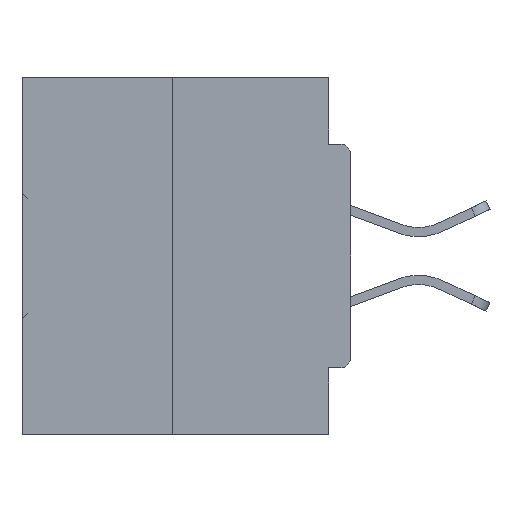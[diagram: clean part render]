
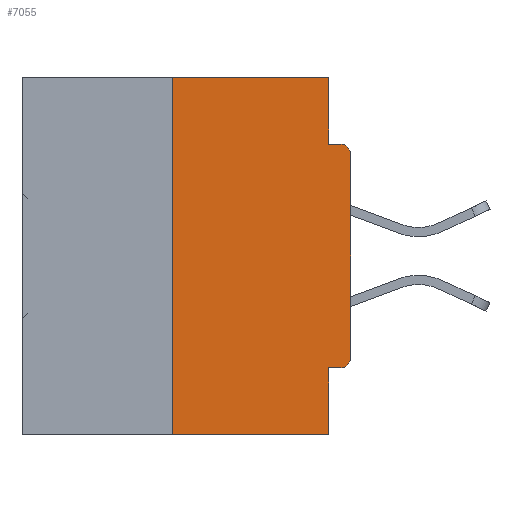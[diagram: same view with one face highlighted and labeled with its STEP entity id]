
A CAD part, left-side view. The second image highlights one B-rep face of the part: STEP entity #7055.
In plain terms, the highlighted planar face has unit normal (-1, 0, 0).
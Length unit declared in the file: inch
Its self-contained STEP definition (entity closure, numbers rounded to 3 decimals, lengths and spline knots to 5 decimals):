
#1575 = VECTOR ( 'NONE', #18556, 39.37008 ) ;
#1924 = DIRECTION ( 'NONE',  ( 0., -1., 0. ) ) ;
#2705 = CARTESIAN_POINT ( 'NONE',  ( 0., 0., 0. ) ) ;
#3144 = VERTEX_POINT ( 'NONE', #39495 ) ;
#3429 = DIRECTION ( 'NONE',  ( -1., 0., 0. ) ) ;
#3908 = EDGE_CURVE ( 'NONE', #16552, #6881, #36625, .T. ) ;
#4827 = VECTOR ( 'NONE', #1924, 39.37008 ) ;
#5094 = ORIENTED_EDGE ( 'NONE', *, *, #28086, .F. ) ;
#5101 = LINE ( 'NONE', #40696, #1575 ) ;
#6521 = VECTOR ( 'NONE', #32120, 39.37008 ) ;
#6881 = VERTEX_POINT ( 'NONE', #27274 ) ;
#7055 = ADVANCED_FACE ( 'NONE', ( #13979 ), #13482, .F. ) ;
#7340 = VECTOR ( 'NONE', #43038, 39.37008 ) ;
#7784 = CARTESIAN_POINT ( 'NONE',  ( 0., 0.015, -0.0935 ) ) ;
#8448 = LINE ( 'NONE', #17828, #7340 ) ;
#8739 = VERTEX_POINT ( 'NONE', #44485 ) ;
#9633 = CARTESIAN_POINT ( 'NONE',  ( 0., 0.46, 0. ) ) ;
#10020 = EDGE_CURVE ( 'NONE', #11931, #46779, #8448, .T. ) ;
#10281 = ORIENTED_EDGE ( 'NONE', *, *, #3908, .T. ) ;
#10805 = EDGE_CURVE ( 'NONE', #3144, #16552, #19893, .T. ) ;
#11190 = CARTESIAN_POINT ( 'NONE',  ( 0., 0.031, -0.5 ) ) ;
#11375 = ORIENTED_EDGE ( 'NONE', *, *, #41169, .F. ) ;
#11489 = EDGE_CURVE ( 'NONE', #29229, #46779, #35936, .T. ) ;
#11931 = VERTEX_POINT ( 'NONE', #34386 ) ;
#13482 = PLANE ( 'NONE',  #47534 ) ;
#13979 = FACE_OUTER_BOUND ( 'NONE', #43682, .T. ) ;
#15105 = CARTESIAN_POINT ( 'NONE',  ( 0., 0.031, -0.5 ) ) ;
#15498 = CARTESIAN_POINT ( 'NONE',  ( 0., 0.015, -0.1085 ) ) ;
#16552 = VERTEX_POINT ( 'NONE', #32540 ) ;
#17175 = DIRECTION ( 'NONE',  ( 1., 0., 0. ) ) ;
#17579 = ORIENTED_EDGE ( 'NONE', *, *, #40966, .F. ) ;
#17828 = CARTESIAN_POINT ( 'NONE',  ( 0., 0.46, -0.5 ) ) ;
#18556 = DIRECTION ( 'NONE',  ( 0., 1., 0. ) ) ;
#18676 = EDGE_CURVE ( 'NONE', #11931, #27597, #25177, .T. ) ;
#19254 = CARTESIAN_POINT ( 'NONE',  ( 0., 0.25, 0. ) ) ;
#19893 = CIRCLE ( 'NONE', #26621, 0.015 ) ;
#20139 = CIRCLE ( 'NONE', #34508, 0.015 ) ;
#20287 = VECTOR ( 'NONE', #37234, 39.37008 ) ;
#23062 = DIRECTION ( 'NONE',  ( 0., 0., -1. ) ) ;
#24182 = EDGE_CURVE ( 'NONE', #6881, #32435, #20139, .T. ) ;
#25177 = LINE ( 'NONE', #41457, #40215 ) ;
#25526 = CARTESIAN_POINT ( 'NONE',  ( 0., 0.015, -0.3915 ) ) ;
#26477 = DIRECTION ( 'NONE',  ( -1., 0., 0. ) ) ;
#26621 = AXIS2_PLACEMENT_3D ( 'NONE', #25526, #3429, #40404 ) ;
#26724 = DIRECTION ( 'NONE',  ( 0., 0., 1. ) ) ;
#27274 = CARTESIAN_POINT ( 'NONE',  ( 0., 0., -0.1085 ) ) ;
#27381 = VERTEX_POINT ( 'NONE', #32079 ) ;
#27597 = VERTEX_POINT ( 'NONE', #19254 ) ;
#28077 = CARTESIAN_POINT ( 'NONE',  ( 0., 0., -0.0935 ) ) ;
#28086 = EDGE_CURVE ( 'NONE', #27597, #8739, #30184, .T. ) ;
#29229 = VERTEX_POINT ( 'NONE', #33260 ) ;
#29304 = VECTOR ( 'NONE', #37919, 39.37008 ) ;
#30184 = LINE ( 'NONE', #42281, #4827 ) ;
#31139 = ORIENTED_EDGE ( 'NONE', *, *, #10805, .T. ) ;
#32079 = CARTESIAN_POINT ( 'NONE',  ( 0., 0.031, -0.0935 ) ) ;
#32120 = DIRECTION ( 'NONE',  ( 0., -1., 0. ) ) ;
#32435 = VERTEX_POINT ( 'NONE', #7784 ) ;
#32540 = CARTESIAN_POINT ( 'NONE',  ( 0., 0., -0.3915 ) ) ;
#33260 = CARTESIAN_POINT ( 'NONE',  ( 0., 0.031, -0.4065 ) ) ;
#33725 = VECTOR ( 'NONE', #36132, 39.37008 ) ;
#34386 = CARTESIAN_POINT ( 'NONE',  ( 0., 0.25, -0.5 ) ) ;
#34508 = AXIS2_PLACEMENT_3D ( 'NONE', #15498, #26477, #23062 ) ;
#34517 = CARTESIAN_POINT ( 'NONE',  ( 0., 0.031, 0. ) ) ;
#34564 = ORIENTED_EDGE ( 'NONE', *, *, #18676, .F. ) ;
#34787 = EDGE_CURVE ( 'NONE', #27381, #32435, #37657, .T. ) ;
#35936 = LINE ( 'NONE', #15105, #20287 ) ;
#36132 = DIRECTION ( 'NONE',  ( 0., 0., 1. ) ) ;
#36625 = LINE ( 'NONE', #2705, #33725 ) ;
#37234 = DIRECTION ( 'NONE',  ( 0., 0., -1. ) ) ;
#37657 = LINE ( 'NONE', #28077, #6521 ) ;
#37919 = DIRECTION ( 'NONE',  ( 0., 0., -1. ) ) ;
#38537 = LINE ( 'NONE', #34517, #29304 ) ;
#39495 = CARTESIAN_POINT ( 'NONE',  ( 0., 0.015, -0.4065 ) ) ;
#40215 = VECTOR ( 'NONE', #26724, 39.37008 ) ;
#40307 = ORIENTED_EDGE ( 'NONE', *, *, #24182, .T. ) ;
#40404 = DIRECTION ( 'NONE',  ( 0., 0., -1. ) ) ;
#40696 = CARTESIAN_POINT ( 'NONE',  ( 0., 0., -0.4065 ) ) ;
#40966 = EDGE_CURVE ( 'NONE', #3144, #29229, #5101, .T. ) ;
#41169 = EDGE_CURVE ( 'NONE', #8739, #27381, #38537, .T. ) ;
#41435 = ORIENTED_EDGE ( 'NONE', *, *, #11489, .F. ) ;
#41457 = CARTESIAN_POINT ( 'NONE',  ( 0., 0.25, 0. ) ) ;
#42281 = CARTESIAN_POINT ( 'NONE',  ( 0., 0.46, 0. ) ) ;
#42696 = DIRECTION ( 'NONE',  ( 0., 0., -1. ) ) ;
#43038 = DIRECTION ( 'NONE',  ( 0., -1., 0. ) ) ;
#43682 = EDGE_LOOP ( 'NONE', ( #5094, #34564, #43729, #41435, #17579, #31139, #10281, #40307, #43908, #11375 ) ) ;
#43729 = ORIENTED_EDGE ( 'NONE', *, *, #10020, .T. ) ;
#43908 = ORIENTED_EDGE ( 'NONE', *, *, #34787, .F. ) ;
#44485 = CARTESIAN_POINT ( 'NONE',  ( 0., 0.031, 0. ) ) ;
#46779 = VERTEX_POINT ( 'NONE', #11190 ) ;
#47534 = AXIS2_PLACEMENT_3D ( 'NONE', #9633, #17175, #42696 ) ;
